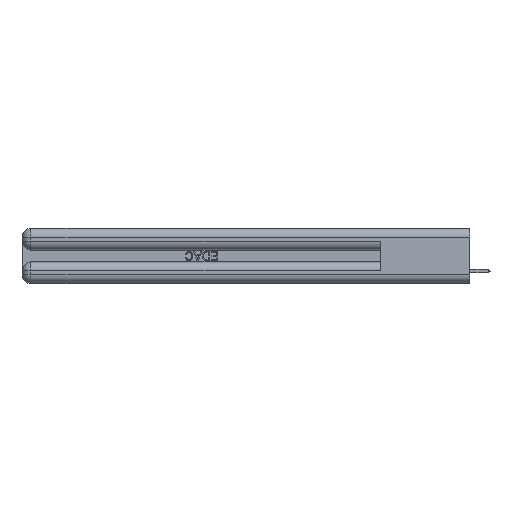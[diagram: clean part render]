
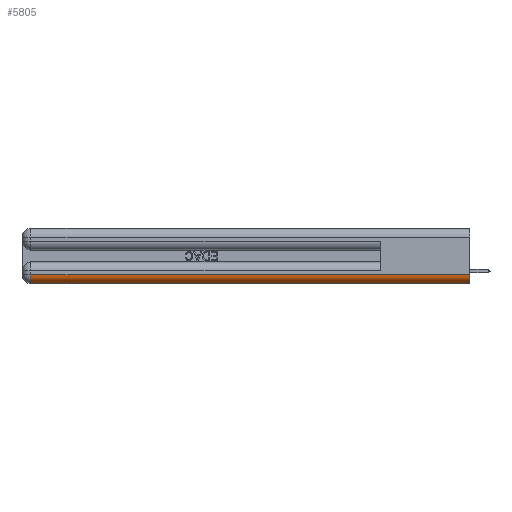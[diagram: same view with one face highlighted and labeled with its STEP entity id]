
A CAD part, left-side view. The second image highlights one B-rep face of the part: STEP entity #5805.
In plain terms, the highlighted cylindrical face has radius 1.524 mm (diameter 3.048 mm), a partial arc.
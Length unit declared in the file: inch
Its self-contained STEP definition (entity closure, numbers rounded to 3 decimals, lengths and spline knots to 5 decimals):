
#119 = VERTEX_POINT ( 'NONE', #24569 ) ;
#370 = ORIENTED_EDGE ( 'NONE', *, *, #28592, .F. ) ;
#1477 = EDGE_CURVE ( 'NONE', #5871, #43502, #40806, .T. ) ;
#2711 = FACE_OUTER_BOUND ( 'NONE', #26369, .T. ) ;
#4140 = AXIS2_PLACEMENT_3D ( 'NONE', #30864, #40956, #31733 ) ;
#5530 = VECTOR ( 'NONE', #12526, 39.37008 ) ;
#5805 = ADVANCED_FACE ( 'NONE', ( #2711 ), #38922, .T. ) ;
#5871 = VERTEX_POINT ( 'NONE', #30396 ) ;
#7555 = ORIENTED_EDGE ( 'NONE', *, *, #1477, .F. ) ;
#12526 = DIRECTION ( 'NONE',  ( 0., -1., 0. ) ) ;
#14468 = AXIS2_PLACEMENT_3D ( 'NONE', #18842, #31920, #32369 ) ;
#16022 = DIRECTION ( 'NONE',  ( 0., 0., 1. ) ) ;
#16308 = DIRECTION ( 'NONE',  ( 0., 1., 0. ) ) ;
#16760 = CARTESIAN_POINT ( 'NONE',  ( 0.06, 2.94, 0. ) ) ;
#17121 = ORIENTED_EDGE ( 'NONE', *, *, #36228, .F. ) ;
#18842 = CARTESIAN_POINT ( 'NONE',  ( 0.06, 0., 0.06 ) ) ;
#22260 = CARTESIAN_POINT ( 'NONE',  ( 0.06, 3., 0. ) ) ;
#22991 = CARTESIAN_POINT ( 'NONE',  ( 0.06, 0., 0.06 ) ) ;
#23673 = LINE ( 'NONE', #29503, #5530 ) ;
#24569 = CARTESIAN_POINT ( 'NONE',  ( 0., 2.94, 0.06 ) ) ;
#26369 = EDGE_LOOP ( 'NONE', ( #31383, #370, #17121, #7555 ) ) ;
#28592 = EDGE_CURVE ( 'NONE', #119, #42059, #23673, .T. ) ;
#28810 = CIRCLE ( 'NONE', #14468, 0.06 ) ;
#29503 = CARTESIAN_POINT ( 'NONE',  ( 0., 0., 0.06 ) ) ;
#30396 = CARTESIAN_POINT ( 'NONE',  ( 0.06, 0., 0. ) ) ;
#30864 = CARTESIAN_POINT ( 'NONE',  ( 0.06, 2.94, 0.06 ) ) ;
#31383 = ORIENTED_EDGE ( 'NONE', *, *, #37662, .F. ) ;
#31733 = DIRECTION ( 'NONE',  ( 0., 0., 1. ) ) ;
#31920 = DIRECTION ( 'NONE',  ( 0., -1., 0. ) ) ;
#32369 = DIRECTION ( 'NONE',  ( 0., 0., 1. ) ) ;
#35617 = DIRECTION ( 'NONE',  ( 0., 1., 0. ) ) ;
#36080 = AXIS2_PLACEMENT_3D ( 'NONE', #22991, #16308, #16022 ) ;
#36228 = EDGE_CURVE ( 'NONE', #43502, #119, #41695, .T. ) ;
#36750 = CARTESIAN_POINT ( 'NONE',  ( 0., 0., 0.06 ) ) ;
#37662 = EDGE_CURVE ( 'NONE', #42059, #5871, #28810, .T. ) ;
#38922 = CYLINDRICAL_SURFACE ( 'NONE', #36080, 0.06 ) ;
#39727 = VECTOR ( 'NONE', #35617, 39.37008 ) ;
#40806 = LINE ( 'NONE', #22260, #39727 ) ;
#40956 = DIRECTION ( 'NONE',  ( 0., 1., 0. ) ) ;
#41695 = CIRCLE ( 'NONE', #4140, 0.06 ) ;
#42059 = VERTEX_POINT ( 'NONE', #36750 ) ;
#43502 = VERTEX_POINT ( 'NONE', #16760 ) ;
